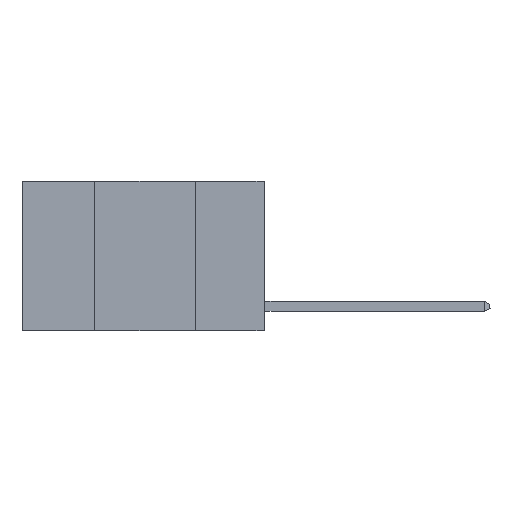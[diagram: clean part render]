
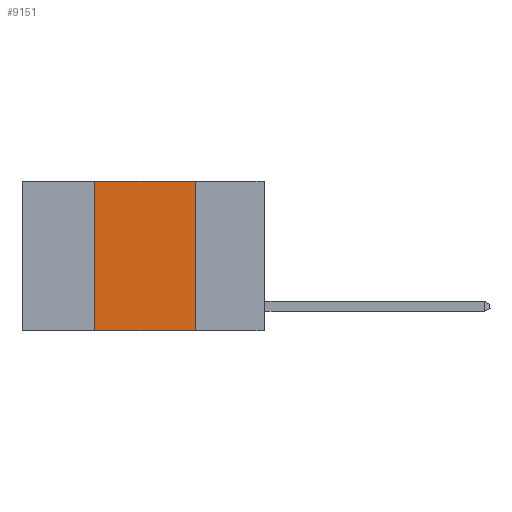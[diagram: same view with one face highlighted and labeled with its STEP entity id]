
A CAD part, left-side view. The second image highlights one B-rep face of the part: STEP entity #9151.
In plain terms, the highlighted planar face has unit normal (-1, 0, 0).
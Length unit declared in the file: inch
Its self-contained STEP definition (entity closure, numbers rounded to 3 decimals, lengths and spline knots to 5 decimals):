
#1 = VECTOR ( 'NONE', #11840, 39.37008 ) ;
#65 = LINE ( 'NONE', #13982, #1 ) ;
#343 = EDGE_CURVE ( 'NONE', #4186, #16608, #9156, .T. ) ;
#537 = CARTESIAN_POINT ( 'NONE',  ( 0., 0.42, -0.37 ) ) ;
#889 = DIRECTION ( 'NONE',  ( 0., -1., 0. ) ) ;
#1622 = ORIENTED_EDGE ( 'NONE', *, *, #11300, .F. ) ;
#3170 = EDGE_CURVE ( 'NONE', #19144, #19304, #65, .T. ) ;
#4186 = VERTEX_POINT ( 'NONE', #7386 ) ;
#4296 = EDGE_LOOP ( 'NONE', ( #20514, #1622, #11302, #8046 ) ) ;
#6030 = VECTOR ( 'NONE', #8754, 39.37008 ) ;
#6304 = CARTESIAN_POINT ( 'NONE',  ( 0., 0.6, 0. ) ) ;
#7386 = CARTESIAN_POINT ( 'NONE',  ( 0., 0.17, 0. ) ) ;
#8009 = FACE_OUTER_BOUND ( 'NONE', #4296, .T. ) ;
#8046 = ORIENTED_EDGE ( 'NONE', *, *, #11668, .T. ) ;
#8754 = DIRECTION ( 'NONE',  ( 0., -1., 0. ) ) ;
#9151 = ADVANCED_FACE ( 'NONE', ( #8009 ), #14625, .F. ) ;
#9156 = LINE ( 'NONE', #16121, #12717 ) ;
#10471 = CARTESIAN_POINT ( 'NONE',  ( 0., 0.6, -0.37 ) ) ;
#11300 = EDGE_CURVE ( 'NONE', #19304, #4186, #16527, .T. ) ;
#11302 = ORIENTED_EDGE ( 'NONE', *, *, #3170, .F. ) ;
#11668 = EDGE_CURVE ( 'NONE', #19144, #16608, #19140, .T. ) ;
#11840 = DIRECTION ( 'NONE',  ( 0., 0., 1. ) ) ;
#12717 = VECTOR ( 'NONE', #14617, 39.37008 ) ;
#13012 = CARTESIAN_POINT ( 'NONE',  ( 0., 0.17, -0.37 ) ) ;
#13266 = DIRECTION ( 'NONE',  ( 1., 0., 0. ) ) ;
#13982 = CARTESIAN_POINT ( 'NONE',  ( 0., 0.42, 0. ) ) ;
#14054 = VECTOR ( 'NONE', #889, 39.37008 ) ;
#14617 = DIRECTION ( 'NONE',  ( 0., 0., -1. ) ) ;
#14625 = PLANE ( 'NONE',  #22299 ) ;
#16121 = CARTESIAN_POINT ( 'NONE',  ( 0., 0.17, 0. ) ) ;
#16527 = LINE ( 'NONE', #16630, #14054 ) ;
#16608 = VERTEX_POINT ( 'NONE', #13012 ) ;
#16630 = CARTESIAN_POINT ( 'NONE',  ( 0., 0.6, 0. ) ) ;
#17085 = CARTESIAN_POINT ( 'NONE',  ( 0., 0.42, 0. ) ) ;
#19140 = LINE ( 'NONE', #10471, #6030 ) ;
#19144 = VERTEX_POINT ( 'NONE', #537 ) ;
#19304 = VERTEX_POINT ( 'NONE', #17085 ) ;
#20215 = DIRECTION ( 'NONE',  ( 0., 0., -1. ) ) ;
#20514 = ORIENTED_EDGE ( 'NONE', *, *, #343, .F. ) ;
#22299 = AXIS2_PLACEMENT_3D ( 'NONE', #6304, #13266, #20215 ) ;
